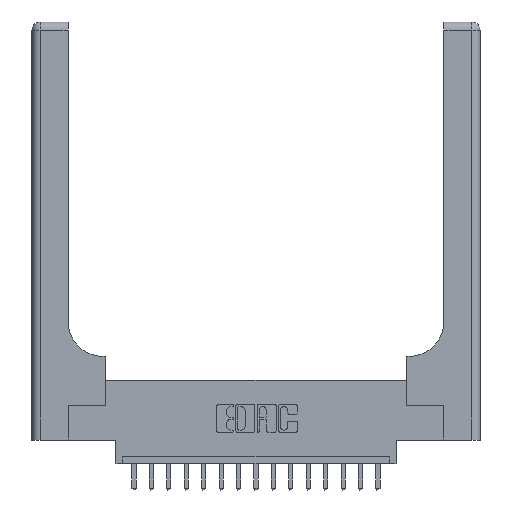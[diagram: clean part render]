
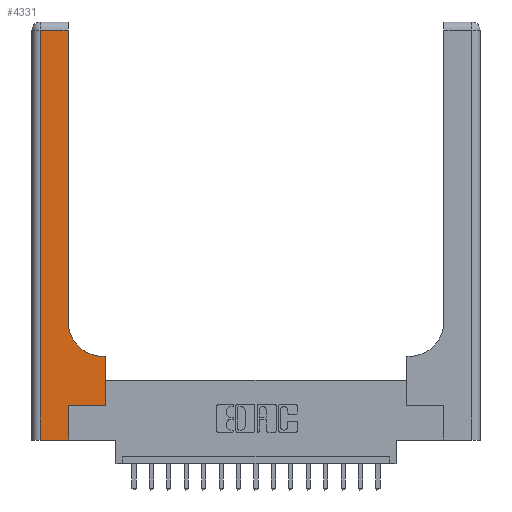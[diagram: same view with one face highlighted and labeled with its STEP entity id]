
A CAD part, top view. The second image highlights one B-rep face of the part: STEP entity #4331.
In plain terms, the highlighted planar face has unit normal (0, 0, 1).
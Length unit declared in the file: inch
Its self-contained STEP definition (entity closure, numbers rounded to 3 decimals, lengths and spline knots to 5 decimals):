
#240 = DIRECTION ( 'NONE',  ( 0., 0., -1. ) ) ;
#290 = DIRECTION ( 'NONE',  ( -1., 0., 0. ) ) ;
#1077 = CARTESIAN_POINT ( 'NONE',  ( 0.06, 3., 0.37 ) ) ;
#1212 = DIRECTION ( 'NONE',  ( 1., 0., 0. ) ) ;
#1220 = DIRECTION ( 'NONE',  ( 0., -1., 0. ) ) ;
#1428 = CARTESIAN_POINT ( 'NONE',  ( 0.265, 0., 0.37 ) ) ;
#2023 = EDGE_CURVE ( 'NONE', #6845, #17940, #11013, .T. ) ;
#2039 = VECTOR ( 'NONE', #9517, 39.37008 ) ;
#2164 = CARTESIAN_POINT ( 'NONE',  ( 0.265, 0.25, 0.37 ) ) ;
#2387 = VECTOR ( 'NONE', #11306, 39.37008 ) ;
#2648 = CARTESIAN_POINT ( 'NONE',  ( 0.528, 0.25, 0.37 ) ) ;
#3038 = CARTESIAN_POINT ( 'NONE',  ( 0., 3., 0.37 ) ) ;
#3417 = VECTOR ( 'NONE', #16170, 39.37008 ) ;
#4331 = ADVANCED_FACE ( 'NONE', ( #11815 ), #5932, .F. ) ;
#4356 = EDGE_LOOP ( 'NONE', ( #17622, #15881, #7244, #4505, #4954, #5047, #7497, #9076, #5259 ) ) ;
#4408 = CARTESIAN_POINT ( 'NONE',  ( 0., 2.94, 0.37 ) ) ;
#4505 = ORIENTED_EDGE ( 'NONE', *, *, #7369, .T. ) ;
#4954 = ORIENTED_EDGE ( 'NONE', *, *, #10116, .T. ) ;
#5020 = VECTOR ( 'NONE', #1220, 39.37008 ) ;
#5047 = ORIENTED_EDGE ( 'NONE', *, *, #17797, .T. ) ;
#5241 = CARTESIAN_POINT ( 'NONE',  ( 0.26, 0.85, 0.37 ) ) ;
#5259 = ORIENTED_EDGE ( 'NONE', *, *, #2023, .T. ) ;
#5548 = VECTOR ( 'NONE', #7230, 39.37008 ) ;
#5932 = PLANE ( 'NONE',  #16828 ) ;
#6281 = LINE ( 'NONE', #12310, #2039 ) ;
#6774 = DIRECTION ( 'NONE',  ( 0., 1., 0. ) ) ;
#6845 = VERTEX_POINT ( 'NONE', #13207 ) ;
#6971 = CARTESIAN_POINT ( 'NONE',  ( 0.51, 0.85, 0.37 ) ) ;
#7230 = DIRECTION ( 'NONE',  ( -1., 0., 0. ) ) ;
#7244 = ORIENTED_EDGE ( 'NONE', *, *, #12342, .T. ) ;
#7369 = EDGE_CURVE ( 'NONE', #10017, #16092, #6281, .T. ) ;
#7382 = CARTESIAN_POINT ( 'NONE',  ( 0.265, 0., 0.37 ) ) ;
#7497 = ORIENTED_EDGE ( 'NONE', *, *, #15383, .T. ) ;
#7500 = LINE ( 'NONE', #1428, #2387 ) ;
#7715 = CARTESIAN_POINT ( 'NONE',  ( 0.528, 0.6, 0.37 ) ) ;
#8089 = EDGE_CURVE ( 'NONE', #17940, #15028, #8875, .T. ) ;
#8252 = LINE ( 'NONE', #16295, #3417 ) ;
#8288 = LINE ( 'NONE', #1077, #5020 ) ;
#8875 = LINE ( 'NONE', #16727, #10643 ) ;
#9076 = ORIENTED_EDGE ( 'NONE', *, *, #14046, .T. ) ;
#9247 = VERTEX_POINT ( 'NONE', #2164 ) ;
#9412 = VERTEX_POINT ( 'NONE', #13871 ) ;
#9517 = DIRECTION ( 'NONE',  ( 1., 0., 0. ) ) ;
#10017 = VERTEX_POINT ( 'NONE', #18015 ) ;
#10116 = EDGE_CURVE ( 'NONE', #16092, #9247, #7500, .T. ) ;
#10643 = VECTOR ( 'NONE', #6774, 39.37008 ) ;
#11013 = CIRCLE ( 'NONE', #14813, 0.25 ) ;
#11306 = DIRECTION ( 'NONE',  ( 0., 1., 0. ) ) ;
#11633 = VERTEX_POINT ( 'NONE', #16721 ) ;
#11815 = FACE_OUTER_BOUND ( 'NONE', #4356, .T. ) ;
#12264 = VERTEX_POINT ( 'NONE', #7715 ) ;
#12305 = VECTOR ( 'NONE', #14827, 39.37008 ) ;
#12310 = CARTESIAN_POINT ( 'NONE',  ( 0., 0., 0.37 ) ) ;
#12342 = EDGE_CURVE ( 'NONE', #9412, #10017, #8288, .T. ) ;
#12642 = VECTOR ( 'NONE', #15493, 39.37008 ) ;
#12985 = LINE ( 'NONE', #13247, #12305 ) ;
#13207 = CARTESIAN_POINT ( 'NONE',  ( 0.51, 0.6, 0.37 ) ) ;
#13247 = CARTESIAN_POINT ( 'NONE',  ( 0.265, 0.25, 0.37 ) ) ;
#13758 = CARTESIAN_POINT ( 'NONE',  ( 0.26, 2.94, 0.37 ) ) ;
#13871 = CARTESIAN_POINT ( 'NONE',  ( 0.06, 2.94, 0.37 ) ) ;
#14046 = EDGE_CURVE ( 'NONE', #12264, #6845, #8252, .T. ) ;
#14813 = AXIS2_PLACEMENT_3D ( 'NONE', #6971, #18326, #1212 ) ;
#14827 = DIRECTION ( 'NONE',  ( 1., 0., 0. ) ) ;
#15028 = VERTEX_POINT ( 'NONE', #13758 ) ;
#15383 = EDGE_CURVE ( 'NONE', #11633, #12264, #17985, .T. ) ;
#15493 = DIRECTION ( 'NONE',  ( 0., 1., 0. ) ) ;
#15881 = ORIENTED_EDGE ( 'NONE', *, *, #17090, .T. ) ;
#16092 = VERTEX_POINT ( 'NONE', #7382 ) ;
#16134 = LINE ( 'NONE', #4408, #5548 ) ;
#16170 = DIRECTION ( 'NONE',  ( -1., 0., 0. ) ) ;
#16295 = CARTESIAN_POINT ( 'NONE',  ( 0.26, 0.6, 0.37 ) ) ;
#16721 = CARTESIAN_POINT ( 'NONE',  ( 0.528, 0.25, 0.37 ) ) ;
#16727 = CARTESIAN_POINT ( 'NONE',  ( 0.26, 3., 0.37 ) ) ;
#16828 = AXIS2_PLACEMENT_3D ( 'NONE', #3038, #240, #290 ) ;
#17090 = EDGE_CURVE ( 'NONE', #15028, #9412, #16134, .T. ) ;
#17622 = ORIENTED_EDGE ( 'NONE', *, *, #8089, .T. ) ;
#17797 = EDGE_CURVE ( 'NONE', #9247, #11633, #12985, .T. ) ;
#17940 = VERTEX_POINT ( 'NONE', #5241 ) ;
#17985 = LINE ( 'NONE', #2648, #12642 ) ;
#18015 = CARTESIAN_POINT ( 'NONE',  ( 0.06, 0., 0.37 ) ) ;
#18326 = DIRECTION ( 'NONE',  ( 0., 0., -1. ) ) ;
